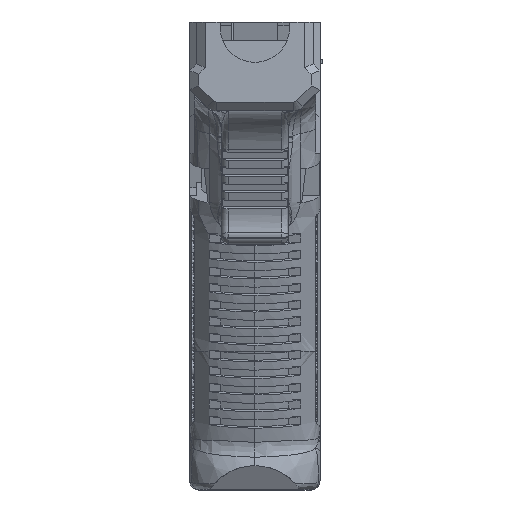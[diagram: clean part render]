
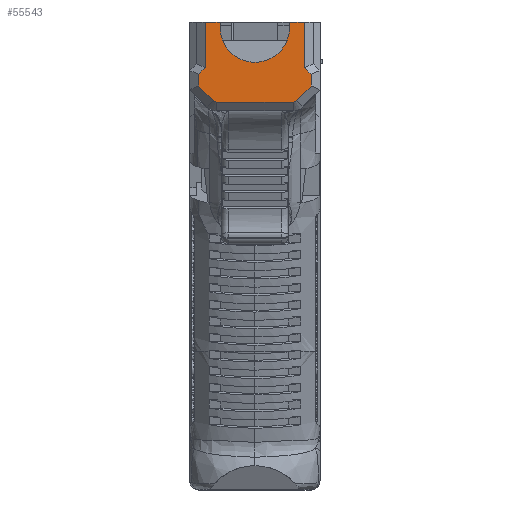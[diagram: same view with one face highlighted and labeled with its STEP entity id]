
A CAD part, left-side view. The second image highlights one B-rep face of the part: STEP entity #55543.
In plain terms, the highlighted planar face has unit normal (-1, 0, 0).
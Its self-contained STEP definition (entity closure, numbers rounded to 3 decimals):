
#6513=PLANE('',#58953);
#7591=LINE('',#66709,#11145);
#7603=LINE('',#66733,#11157);
#7723=LINE('',#67561,#11277);
#7725=LINE('',#67565,#11279);
#7726=LINE('',#67568,#11280);
#7727=LINE('',#67570,#11281);
#7728=LINE('',#67572,#11282);
#7729=LINE('',#67574,#11283);
#7730=LINE('',#67576,#11284);
#7731=LINE('',#67583,#11285);
#7732=LINE('',#67590,#11286);
#7733=LINE('',#67592,#11287);
#7734=LINE('',#67593,#11288);
#11145=VECTOR('',#60421,10.);
#11157=VECTOR('',#60435,10.);
#11277=VECTOR('',#60599,10.);
#11279=VECTOR('',#60603,10.);
#11280=VECTOR('',#60606,10.);
#11281=VECTOR('',#60607,10.);
#11282=VECTOR('',#60608,10.);
#11283=VECTOR('',#60609,10.);
#11284=VECTOR('',#60610,10.);
#11285=VECTOR('',#60611,10.);
#11286=VECTOR('',#60612,10.);
#11287=VECTOR('',#60613,10.);
#11288=VECTOR('',#60614,10.);
#14737=FACE_OUTER_BOUND('',#18115,.T.);
#18115=EDGE_LOOP('',(#38301,#38302,#38303,#38304,#38305,#38306,#38307,#38308,
#38309,#38310,#38311,#38312,#38313,#38314,#38315,#38316));
#21878=CIRCLE('',#58954,7.765);
#22073=B_SPLINE_CURVE_WITH_KNOTS('',3,(#67578,#67579,#67580,#67581),
 .UNSPECIFIED.,.F.,.F.,(4,4),(-0.393,0.393),
 .UNSPECIFIED.);
#22074=B_SPLINE_CURVE_WITH_KNOTS('',3,(#67585,#67586,#67587,#67588),
 .UNSPECIFIED.,.F.,.F.,(4,4),(-0.393,0.393),
 .UNSPECIFIED.);
#23389=VERTEX_POINT('',#66706);
#23390=VERTEX_POINT('',#66708);
#23400=VERTEX_POINT('',#66730);
#23401=VERTEX_POINT('',#66732);
#23555=VERTEX_POINT('',#67560);
#23556=VERTEX_POINT('',#67564);
#23557=VERTEX_POINT('',#67566);
#23558=VERTEX_POINT('',#67569);
#23559=VERTEX_POINT('',#67571);
#23560=VERTEX_POINT('',#67573);
#23561=VERTEX_POINT('',#67575);
#23562=VERTEX_POINT('',#67577);
#23563=VERTEX_POINT('',#67582);
#23564=VERTEX_POINT('',#67584);
#23565=VERTEX_POINT('',#67589);
#23566=VERTEX_POINT('',#67591);
#29236=EDGE_CURVE('',#23390,#23389,#7591,.T.);
#29248=EDGE_CURVE('',#23401,#23400,#7603,.T.);
#29417=EDGE_CURVE('',#23401,#23555,#7723,.T.);
#29419=EDGE_CURVE('',#23400,#23556,#7725,.T.);
#29420=EDGE_CURVE('',#23556,#23557,#21878,.T.);
#29421=EDGE_CURVE('',#23557,#23390,#7726,.T.);
#29422=EDGE_CURVE('',#23558,#23389,#7727,.T.);
#29423=EDGE_CURVE('',#23559,#23558,#7728,.T.);
#29424=EDGE_CURVE('',#23560,#23559,#7729,.T.);
#29425=EDGE_CURVE('',#23561,#23560,#7730,.T.);
#29426=EDGE_CURVE('',#23562,#23561,#22073,.T.);
#29427=EDGE_CURVE('',#23563,#23562,#7731,.T.);
#29428=EDGE_CURVE('',#23564,#23563,#22074,.T.);
#29429=EDGE_CURVE('',#23565,#23564,#7732,.T.);
#29430=EDGE_CURVE('',#23566,#23565,#7733,.T.);
#29431=EDGE_CURVE('',#23555,#23566,#7734,.T.);
#38301=ORIENTED_EDGE('',*,*,#29248,.T.);
#38302=ORIENTED_EDGE('',*,*,#29419,.T.);
#38303=ORIENTED_EDGE('',*,*,#29420,.T.);
#38304=ORIENTED_EDGE('',*,*,#29421,.T.);
#38305=ORIENTED_EDGE('',*,*,#29236,.T.);
#38306=ORIENTED_EDGE('',*,*,#29422,.F.);
#38307=ORIENTED_EDGE('',*,*,#29423,.F.);
#38308=ORIENTED_EDGE('',*,*,#29424,.F.);
#38309=ORIENTED_EDGE('',*,*,#29425,.F.);
#38310=ORIENTED_EDGE('',*,*,#29426,.F.);
#38311=ORIENTED_EDGE('',*,*,#29427,.F.);
#38312=ORIENTED_EDGE('',*,*,#29428,.F.);
#38313=ORIENTED_EDGE('',*,*,#29429,.F.);
#38314=ORIENTED_EDGE('',*,*,#29430,.F.);
#38315=ORIENTED_EDGE('',*,*,#29431,.F.);
#38316=ORIENTED_EDGE('',*,*,#29417,.F.);
#55543=ADVANCED_FACE('',(#14737),#6513,.F.);
#58953=AXIS2_PLACEMENT_3D('',#67563,#60601,#60602);
#58954=AXIS2_PLACEMENT_3D('',#67567,#60604,#60605);
#60421=DIRECTION('',(0.,1.,0.));
#60435=DIRECTION('',(0.,1.,0.));
#60599=DIRECTION('',(0.,0.,-1.));
#60601=DIRECTION('center_axis',(1.,0.,
0.));
#60602=DIRECTION('ref_axis',(0.,1.,0.));
#60603=DIRECTION('',(0.,0.,-1.));
#60604=DIRECTION('center_axis',(1.,0.,
0.));
#60605=DIRECTION('ref_axis',(0.,0.,
-1.));
#60606=DIRECTION('',(0.,0.,1.));
#60607=DIRECTION('',(0.,0.,1.));
#60608=DIRECTION('',(0.,-0.707,0.707));
#60609=DIRECTION('',(0.,0.,1.));
#60610=DIRECTION('',(0.,0.707,0.707));
#60611=DIRECTION('',(0.,1.,0.));
#60612=DIRECTION('',(0.,0.707,-0.707));
#60613=DIRECTION('',(0.,0.,-1.));
#60614=DIRECTION('',(0.,-0.707,-0.707));
#66706=CARTESIAN_POINT('',(107.368,-4.034,-24.061));
#66708=CARTESIAN_POINT('',(107.368,-7.386,-24.061));
#66709=CARTESIAN_POINT('',(107.368,-22.763,-24.061));
#66730=CARTESIAN_POINT('',(107.368,-22.914,-24.061));
#66732=CARTESIAN_POINT('',(107.368,-26.266,-24.061));
#66733=CARTESIAN_POINT('',(107.368,-22.763,-24.061));
#67560=CARTESIAN_POINT('',(107.368,-26.266,-34.275));
#67561=CARTESIAN_POINT('',(107.368,-26.266,-55.047));
#67563=CARTESIAN_POINT('Origin',(107.367,-15.151,-76.647));
#67564=CARTESIAN_POINT('',(107.368,-22.914,-25.477));
#67565=CARTESIAN_POINT('',(107.368,-22.914,-50.935));
#67566=CARTESIAN_POINT('',(107.368,-7.386,-25.477));
#67567=CARTESIAN_POINT('Origin',(107.368,-15.15,-25.35));
#67568=CARTESIAN_POINT('',(107.368,-7.386,-50.935));
#67569=CARTESIAN_POINT('',(107.368,-4.034,-34.275));
#67570=CARTESIAN_POINT('',(107.368,-4.034,-50.047));
#67571=CARTESIAN_POINT('',(107.368,-2.534,-35.775));
#67572=CARTESIAN_POINT('',(107.368,4.448,-42.757));
#67573=CARTESIAN_POINT('',(107.368,-2.534,-38.422));
#67574=CARTESIAN_POINT('',(107.368,-2.534,-50.301));
#67575=CARTESIAN_POINT('',(107.368,-5.819,-41.708));
#67576=CARTESIAN_POINT('',(107.368,-16.139,-52.027));
#67577=CARTESIAN_POINT('',(107.368,-6.527,-42.));
#67578=CARTESIAN_POINT('Ctrl Pts',(107.368,-6.527,-42.));
#67579=CARTESIAN_POINT('Ctrl Pts',(107.368,-6.265,-42.));
#67580=CARTESIAN_POINT('Ctrl Pts',(107.368,-6.005,-41.893));
#67581=CARTESIAN_POINT('Ctrl Pts',(107.368,-5.819,-41.708));
#67582=CARTESIAN_POINT('',(107.368,-23.773,-42.));
#67583=CARTESIAN_POINT('',(107.368,-15.15,-42.));
#67584=CARTESIAN_POINT('',(107.368,-24.48,-41.708));
#67585=CARTESIAN_POINT('Ctrl Pts',(107.368,-24.48,-41.708));
#67586=CARTESIAN_POINT('Ctrl Pts',(107.368,-24.295,-41.893));
#67587=CARTESIAN_POINT('Ctrl Pts',(107.368,-24.035,-42.));
#67588=CARTESIAN_POINT('Ctrl Pts',(107.368,-23.773,-42.));
#67589=CARTESIAN_POINT('',(107.368,-27.766,-38.422));
#67590=CARTESIAN_POINT('',(107.368,-14.161,-52.027));
#67591=CARTESIAN_POINT('',(107.368,-27.766,-35.775));
#67592=CARTESIAN_POINT('',(107.368,-27.766,-50.301));
#67593=CARTESIAN_POINT('',(107.368,-34.748,-42.757));
